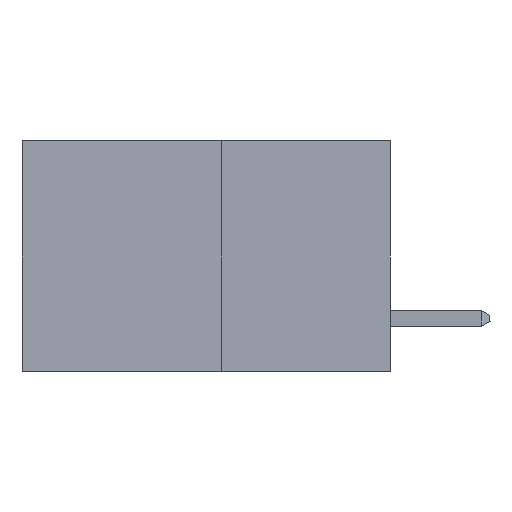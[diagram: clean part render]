
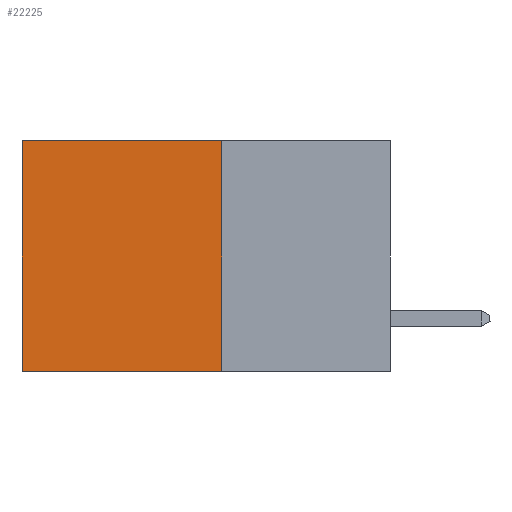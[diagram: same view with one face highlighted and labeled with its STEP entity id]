
A CAD part, left-side view. The second image highlights one B-rep face of the part: STEP entity #22225.
In plain terms, the highlighted planar face has unit normal (-1, 0, 0).
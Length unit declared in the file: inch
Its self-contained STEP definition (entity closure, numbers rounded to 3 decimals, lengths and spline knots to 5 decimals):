
#543 = ORIENTED_EDGE ( 'NONE', *, *, #20765, .F. ) ;
#1113 = EDGE_CURVE ( 'NONE', #18588, #17758, #17647, .T. ) ;
#1272 = LINE ( 'NONE', #21461, #15306 ) ;
#2159 = VECTOR ( 'NONE', #21667, 39.37008 ) ;
#2822 = CARTESIAN_POINT ( 'NONE',  ( 0.277, 0.59, 0. ) ) ;
#3127 = VECTOR ( 'NONE', #12530, 39.37008 ) ;
#3254 = EDGE_CURVE ( 'NONE', #17758, #6883, #7012, .T. ) ;
#3336 = FACE_OUTER_BOUND ( 'NONE', #14496, .T. ) ;
#3415 = CARTESIAN_POINT ( 'NONE',  ( 0.277, 0.27, 0. ) ) ;
#4878 = VERTEX_POINT ( 'NONE', #18347 ) ;
#5479 = AXIS2_PLACEMENT_3D ( 'NONE', #9250, #21984, #11106 ) ;
#5717 = CARTESIAN_POINT ( 'NONE',  ( 0.277, 0.27, 0. ) ) ;
#6883 = VERTEX_POINT ( 'NONE', #22095 ) ;
#6890 = DIRECTION ( 'NONE',  ( 0., 1., 0. ) ) ;
#6978 = CARTESIAN_POINT ( 'NONE',  ( 0.277, 0.27, -0.37 ) ) ;
#7012 = LINE ( 'NONE', #14373, #2159 ) ;
#7958 = VECTOR ( 'NONE', #18695, 39.37008 ) ;
#8568 = LINE ( 'NONE', #6978, #3127 ) ;
#9250 = CARTESIAN_POINT ( 'NONE',  ( 0.277, 0.27, -0.37 ) ) ;
#11020 = PLANE ( 'NONE',  #5479 ) ;
#11106 = DIRECTION ( 'NONE',  ( 0., 0., -1. ) ) ;
#12530 = DIRECTION ( 'NONE',  ( 0., 0., -1. ) ) ;
#13718 = ORIENTED_EDGE ( 'NONE', *, *, #3254, .T. ) ;
#14149 = ORIENTED_EDGE ( 'NONE', *, *, #23392, .F. ) ;
#14373 = CARTESIAN_POINT ( 'NONE',  ( 0.277, 0.59, -0.37 ) ) ;
#14496 = EDGE_LOOP ( 'NONE', ( #13718, #14149, #543, #21748 ) ) ;
#15306 = VECTOR ( 'NONE', #6890, 39.37008 ) ;
#17647 = LINE ( 'NONE', #5717, #7958 ) ;
#17758 = VERTEX_POINT ( 'NONE', #2822 ) ;
#18347 = CARTESIAN_POINT ( 'NONE',  ( 0.277, 0.27, -0.37 ) ) ;
#18588 = VERTEX_POINT ( 'NONE', #3415 ) ;
#18695 = DIRECTION ( 'NONE',  ( 0., 1., 0. ) ) ;
#20765 = EDGE_CURVE ( 'NONE', #18588, #4878, #8568, .T. ) ;
#21461 = CARTESIAN_POINT ( 'NONE',  ( 0.277, 0.27, -0.37 ) ) ;
#21667 = DIRECTION ( 'NONE',  ( 0., 0., -1. ) ) ;
#21748 = ORIENTED_EDGE ( 'NONE', *, *, #1113, .T. ) ;
#21984 = DIRECTION ( 'NONE',  ( 1., 0., 0. ) ) ;
#22095 = CARTESIAN_POINT ( 'NONE',  ( 0.277, 0.59, -0.37 ) ) ;
#22225 = ADVANCED_FACE ( 'NONE', ( #3336 ), #11020, .F. ) ;
#23392 = EDGE_CURVE ( 'NONE', #4878, #6883, #1272, .T. ) ;
